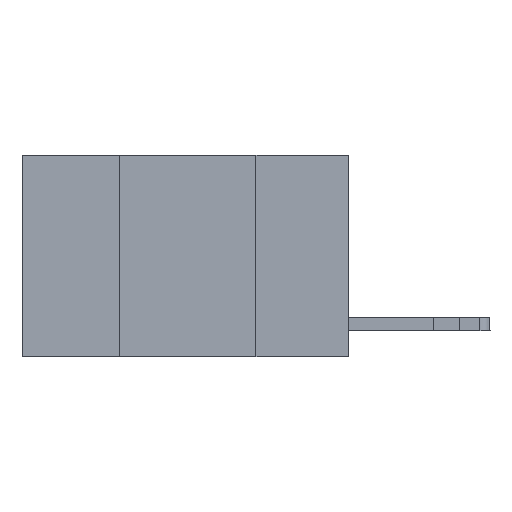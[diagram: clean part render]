
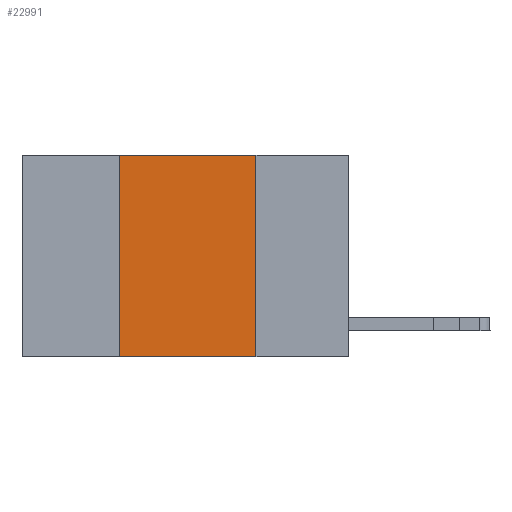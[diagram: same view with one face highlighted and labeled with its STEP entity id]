
A CAD part, left-side view. The second image highlights one B-rep face of the part: STEP entity #22991.
In plain terms, the highlighted planar face has unit normal (-1, 0, 0).
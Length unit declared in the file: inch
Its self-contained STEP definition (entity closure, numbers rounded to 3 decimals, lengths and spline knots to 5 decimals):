
#301 = ORIENTED_EDGE ( 'NONE', *, *, #17771, .F. ) ;
#1390 = ORIENTED_EDGE ( 'NONE', *, *, #5193, .F. ) ;
#1906 = ORIENTED_EDGE ( 'NONE', *, *, #20728, .T. ) ;
#2252 = PLANE ( 'NONE',  #6409 ) ;
#2557 = VERTEX_POINT ( 'NONE', #8279 ) ;
#3076 = LINE ( 'NONE', #21943, #14783 ) ;
#5193 = EDGE_CURVE ( 'NONE', #18227, #17831, #13995, .T. ) ;
#5613 = FACE_OUTER_BOUND ( 'NONE', #16934, .T. ) ;
#6409 = AXIS2_PLACEMENT_3D ( 'NONE', #18811, #7804, #14819 ) ;
#7235 = DIRECTION ( 'NONE',  ( 0., -1., 0. ) ) ;
#7804 = DIRECTION ( 'NONE',  ( 1., 0., 0. ) ) ;
#8279 = CARTESIAN_POINT ( 'NONE',  ( 0., 0.17, 0. ) ) ;
#9051 = EDGE_CURVE ( 'NONE', #17831, #2557, #19498, .T. ) ;
#9717 = VECTOR ( 'NONE', #7235, 39.37008 ) ;
#10428 = DIRECTION ( 'NONE',  ( 0., 0., -1. ) ) ;
#10812 = CARTESIAN_POINT ( 'NONE',  ( 0., 0.17, -0.37 ) ) ;
#11022 = CARTESIAN_POINT ( 'NONE',  ( 0., 0.42, 0. ) ) ;
#11345 = CARTESIAN_POINT ( 'NONE',  ( 0., 0.42, -0.37 ) ) ;
#13426 = CARTESIAN_POINT ( 'NONE',  ( 0., 0.42, 0. ) ) ;
#13523 = LINE ( 'NONE', #15104, #14454 ) ;
#13995 = LINE ( 'NONE', #13426, #23515 ) ;
#14117 = DIRECTION ( 'NONE',  ( 0., 0., 1. ) ) ;
#14454 = VECTOR ( 'NONE', #20688, 39.37008 ) ;
#14557 = VERTEX_POINT ( 'NONE', #10812 ) ;
#14783 = VECTOR ( 'NONE', #10428, 39.37008 ) ;
#14819 = DIRECTION ( 'NONE',  ( 0., 0., -1. ) ) ;
#15104 = CARTESIAN_POINT ( 'NONE',  ( 0., 0.6, -0.37 ) ) ;
#15847 = CARTESIAN_POINT ( 'NONE',  ( 0., 0.6, 0. ) ) ;
#16934 = EDGE_LOOP ( 'NONE', ( #301, #20433, #1390, #1906 ) ) ;
#17771 = EDGE_CURVE ( 'NONE', #2557, #14557, #3076, .T. ) ;
#17831 = VERTEX_POINT ( 'NONE', #11022 ) ;
#18227 = VERTEX_POINT ( 'NONE', #11345 ) ;
#18811 = CARTESIAN_POINT ( 'NONE',  ( 0., 0.6, 0. ) ) ;
#19498 = LINE ( 'NONE', #15847, #9717 ) ;
#20433 = ORIENTED_EDGE ( 'NONE', *, *, #9051, .F. ) ;
#20688 = DIRECTION ( 'NONE',  ( 0., -1., 0. ) ) ;
#20728 = EDGE_CURVE ( 'NONE', #18227, #14557, #13523, .T. ) ;
#21943 = CARTESIAN_POINT ( 'NONE',  ( 0., 0.17, 0. ) ) ;
#22991 = ADVANCED_FACE ( 'NONE', ( #5613 ), #2252, .F. ) ;
#23515 = VECTOR ( 'NONE', #14117, 39.37008 ) ;
